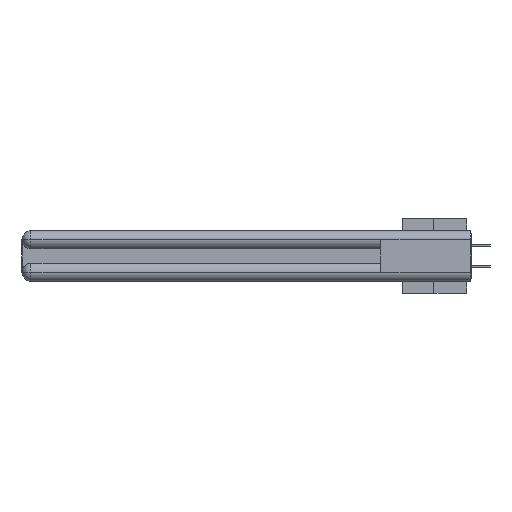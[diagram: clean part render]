
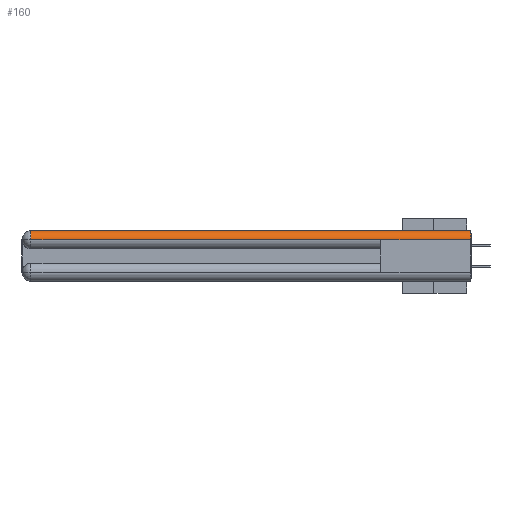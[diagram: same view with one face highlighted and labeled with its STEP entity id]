
A CAD part, left-side view. The second image highlights one B-rep face of the part: STEP entity #160.
In plain terms, the highlighted cylindrical face has radius 1.562 mm (diameter 3.124 mm), a partial arc.
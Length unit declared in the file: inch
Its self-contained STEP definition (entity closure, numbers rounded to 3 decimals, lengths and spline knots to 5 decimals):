
#160 = ADVANCED_FACE ( 'NONE', ( #3368 ), #24109, .T. ) ;
#951 = CARTESIAN_POINT ( 'NONE',  ( 0., 2.94, -0.0615 ) ) ;
#1650 = CARTESIAN_POINT ( 'NONE',  ( 0.0615, 0., -0.0615 ) ) ;
#3007 = EDGE_CURVE ( 'NONE', #18184, #19978, #13529, .T. ) ;
#3368 = FACE_OUTER_BOUND ( 'NONE', #17805, .T. ) ;
#4019 = ORIENTED_EDGE ( 'NONE', *, *, #41467, .F. ) ;
#4645 = ORIENTED_EDGE ( 'NONE', *, *, #3007, .F. ) ;
#4726 = CARTESIAN_POINT ( 'NONE',  ( 0., 3., -0.0615 ) ) ;
#5623 = EDGE_CURVE ( 'NONE', #39911, #35085, #27064, .T. ) ;
#6916 = DIRECTION ( 'NONE',  ( 0., 0., 1. ) ) ;
#10199 = DIRECTION ( 'NONE',  ( 0., -1., 0. ) ) ;
#10396 = ORIENTED_EDGE ( 'NONE', *, *, #42092, .F. ) ;
#11308 = VECTOR ( 'NONE', #37240, 39.37008 ) ;
#12736 = CARTESIAN_POINT ( 'NONE',  ( 0., 3., -0.0615 ) ) ;
#12758 = CARTESIAN_POINT ( 'NONE',  ( 0.0615, 0., -0.0615 ) ) ;
#13204 = CARTESIAN_POINT ( 'NONE',  ( 0.0615, 2.94, -0.0615 ) ) ;
#13529 = LINE ( 'NONE', #39194, #24427 ) ;
#15389 = ORIENTED_EDGE ( 'NONE', *, *, #5623, .T. ) ;
#15403 = DIRECTION ( 'NONE',  ( 0., -1., 0. ) ) ;
#16532 = DIRECTION ( 'NONE',  ( 0., -1., 0. ) ) ;
#17805 = EDGE_LOOP ( 'NONE', ( #4645, #38208, #15389, #10396, #4019 ) ) ;
#18184 = VERTEX_POINT ( 'NONE', #31346 ) ;
#19978 = VERTEX_POINT ( 'NONE', #44714 ) ;
#20604 = CIRCLE ( 'NONE', #41493, 0.0615 ) ;
#21081 = AXIS2_PLACEMENT_3D ( 'NONE', #1650, #15403, #26164 ) ;
#24109 = CYLINDRICAL_SURFACE ( 'NONE', #42014, 0.0615 ) ;
#24427 = VECTOR ( 'NONE', #10199, 39.37008 ) ;
#26164 = DIRECTION ( 'NONE',  ( 1., 0., 0. ) ) ;
#26585 = DIRECTION ( 'NONE',  ( 0., 1., 0. ) ) ;
#26860 = LINE ( 'NONE', #4726, #32895 ) ;
#27064 = LINE ( 'NONE', #12736, #11308 ) ;
#30317 = CARTESIAN_POINT ( 'NONE',  ( 0., 0.6, -0.0615 ) ) ;
#30538 = VERTEX_POINT ( 'NONE', #34379 ) ;
#31346 = CARTESIAN_POINT ( 'NONE',  ( 0.0615, 2.94, 0. ) ) ;
#32895 = VECTOR ( 'NONE', #42891, 39.37008 ) ;
#34379 = CARTESIAN_POINT ( 'NONE',  ( 0., 0., -0.0615 ) ) ;
#35085 = VERTEX_POINT ( 'NONE', #30317 ) ;
#37240 = DIRECTION ( 'NONE',  ( 0., -1., 0. ) ) ;
#38208 = ORIENTED_EDGE ( 'NONE', *, *, #43668, .T. ) ;
#39194 = CARTESIAN_POINT ( 'NONE',  ( 0.0615, 0., 0. ) ) ;
#39911 = VERTEX_POINT ( 'NONE', #951 ) ;
#40009 = CIRCLE ( 'NONE', #21081, 0.0615 ) ;
#40878 = DIRECTION ( 'NONE',  ( 0., 0., 1. ) ) ;
#41467 = EDGE_CURVE ( 'NONE', #19978, #30538, #40009, .T. ) ;
#41493 = AXIS2_PLACEMENT_3D ( 'NONE', #13204, #16532, #40878 ) ;
#42014 = AXIS2_PLACEMENT_3D ( 'NONE', #12758, #26585, #6916 ) ;
#42092 = EDGE_CURVE ( 'NONE', #30538, #35085, #26860, .T. ) ;
#42891 = DIRECTION ( 'NONE',  ( 0., 1., 0. ) ) ;
#43668 = EDGE_CURVE ( 'NONE', #18184, #39911, #20604, .T. ) ;
#44714 = CARTESIAN_POINT ( 'NONE',  ( 0.0615, 0., 0. ) ) ;
